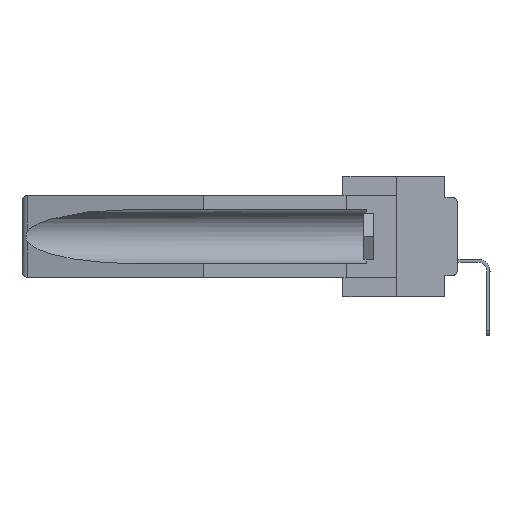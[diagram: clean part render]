
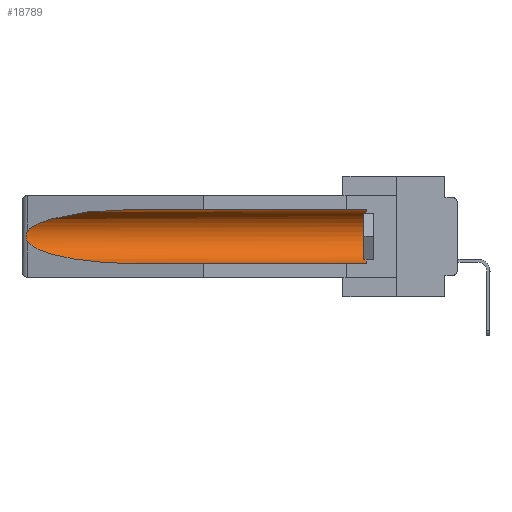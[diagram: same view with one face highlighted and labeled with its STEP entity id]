
A CAD part, left-side view. The second image highlights one B-rep face of the part: STEP entity #18789.
In plain terms, the highlighted cylindrical face has radius 2.857 mm (diameter 5.715 mm), a partial arc.
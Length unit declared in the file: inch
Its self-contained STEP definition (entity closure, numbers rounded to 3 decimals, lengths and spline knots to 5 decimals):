
#248 = DIRECTION ( 'NONE',  ( 0., 1., 0. ) ) ;
#819 = DIRECTION ( 'NONE',  ( 0., -1., 0. ) ) ;
#1037 = ORIENTED_EDGE ( 'NONE', *, *, #22426, .T. ) ;
#1324 = VECTOR ( 'NONE', #248, 39.37008 ) ;
#1703 = EDGE_LOOP ( 'NONE', ( #1764, #1037, #18259, #5178, #1854, #29031 ) ) ;
#1764 = ORIENTED_EDGE ( 'NONE', *, *, #3592, .T. ) ;
#1811 = CARTESIAN_POINT ( 'NONE',  ( 0.26537, 1.52718, -0.14972 ) ) ;
#1854 = ORIENTED_EDGE ( 'NONE', *, *, #24292, .T. ) ;
#1892 = AXIS2_PLACEMENT_3D ( 'NONE', #28931, #8678, #13623 ) ;
#2769 =( BOUNDED_CURVE ( )  B_SPLINE_CURVE ( 3, ( #29566, #17259, #4664, #7214 ),
 .UNSPECIFIED., .F., .F. ) 
 B_SPLINE_CURVE_WITH_KNOTS ( ( 4, 4 ),
 ( 0.1948, 1.5708 ),
 .UNSPECIFIED. ) 
 CURVE ( )  GEOMETRIC_REPRESENTATION_ITEM ( )  RATIONAL_B_SPLINE_CURVE ( ( 1., 0.848, 0.848, 1. ) ) 
 REPRESENTATION_ITEM ( '' )  );
#2864 = CARTESIAN_POINT ( 'NONE',  ( 0.26597, 1.52961, -0.15275 ) ) ;
#2960 = CARTESIAN_POINT ( 'NONE',  ( 0.2675, 1.53308, -0.17534 ) ) ;
#3379 = CARTESIAN_POINT ( 'NONE',  ( 0.26537, 1.52718, -0.14972 ) ) ;
#3592 = EDGE_CURVE ( 'NONE', #9058, #27754, #6649, .T. ) ;
#3792 = CARTESIAN_POINT ( 'NONE',  ( 0.2673, 1.53269, -0.17917 ) ) ;
#4254 = CARTESIAN_POINT ( 'NONE',  ( 0.155, 1.07973, -0.059 ) ) ;
#4664 = CARTESIAN_POINT ( 'NONE',  ( 0.21114, 1.30732, -0.284 ) ) ;
#4890 = CYLINDRICAL_SURFACE ( 'NONE', #1892, 0.1125 ) ;
#5091 = CIRCLE ( 'NONE', #12571, 0.1125 ) ;
#5178 = ORIENTED_EDGE ( 'NONE', *, *, #19157, .F. ) ;
#6057 = CARTESIAN_POINT ( 'NONE',  ( 0.155, 0.126, -0.1715 ) ) ;
#6424 = VERTEX_POINT ( 'NONE', #31843 ) ;
#6649 =( BOUNDED_CURVE ( )  B_SPLINE_CURVE ( 3, ( #4254, #21891, #22114, #1811 ),
 .UNSPECIFIED., .F., .F. ) 
 B_SPLINE_CURVE_WITH_KNOTS ( ( 4, 4 ),
 ( 4.71239, 6.08839 ),
 .UNSPECIFIED. ) 
 CURVE ( )  GEOMETRIC_REPRESENTATION_ITEM ( )  RATIONAL_B_SPLINE_CURVE ( ( 1., 0.848, 0.848, 1. ) ) 
 REPRESENTATION_ITEM ( '' )  );
#7214 = CARTESIAN_POINT ( 'NONE',  ( 0.155, 1.07973, -0.284 ) ) ;
#8256 = B_SPLINE_CURVE_WITH_KNOTS ( 'NONE', 3,
 ( #22686, #2864, #20324, #20540, #13003, #2960, #3792, #9309, #13583, #29938 ),
 .UNSPECIFIED., .F., .F.,
 ( 4, 2, 2, 2, 4 ),
 ( 0., 0.00029, 0.00058, 0.00087, 0.00117 ),
 .UNSPECIFIED. ) ;
#8678 = DIRECTION ( 'NONE',  ( 0., 1., 0. ) ) ;
#9058 = VERTEX_POINT ( 'NONE', #22231 ) ;
#9250 = CARTESIAN_POINT ( 'NONE',  ( 0.155, -0.30754, -0.059 ) ) ;
#9309 = CARTESIAN_POINT ( 'NONE',  ( 0.26655, 1.53094, -0.18657 ) ) ;
#9631 = LINE ( 'NONE', #12727, #1324 ) ;
#12571 = AXIS2_PLACEMENT_3D ( 'NONE', #6057, #819, #13618 ) ;
#12727 = CARTESIAN_POINT ( 'NONE',  ( 0.155, -0.30754, -0.284 ) ) ;
#13003 = CARTESIAN_POINT ( 'NONE',  ( 0.2675, 1.53308, -0.16763 ) ) ;
#13583 = CARTESIAN_POINT ( 'NONE',  ( 0.26597, 1.5296, -0.19026 ) ) ;
#13618 = DIRECTION ( 'NONE',  ( 0., 0., 1. ) ) ;
#13623 = DIRECTION ( 'NONE',  ( 0., 0., 1. ) ) ;
#13958 = FACE_OUTER_BOUND ( 'NONE', #1703, .T. ) ;
#17007 = CARTESIAN_POINT ( 'NONE',  ( 0.155, 0.126, -0.284 ) ) ;
#17259 = CARTESIAN_POINT ( 'NONE',  ( 0.25451, 1.48313, -0.24835 ) ) ;
#18259 = ORIENTED_EDGE ( 'NONE', *, *, #26882, .T. ) ;
#18296 = VERTEX_POINT ( 'NONE', #17007 ) ;
#18789 = ADVANCED_FACE ( 'NONE', ( #13958 ), #4890, .F. ) ;
#19157 = EDGE_CURVE ( 'NONE', #18296, #25073, #9631, .T. ) ;
#19195 = VERTEX_POINT ( 'NONE', #25517 ) ;
#19422 = DIRECTION ( 'NONE',  ( 0., 1., 0. ) ) ;
#19493 = EDGE_CURVE ( 'NONE', #6424, #9058, #23428, .T. ) ;
#20324 = CARTESIAN_POINT ( 'NONE',  ( 0.26654, 1.53092, -0.15636 ) ) ;
#20540 = CARTESIAN_POINT ( 'NONE',  ( 0.2673, 1.5327, -0.16383 ) ) ;
#21891 = CARTESIAN_POINT ( 'NONE',  ( 0.21114, 1.30732, -0.059 ) ) ;
#22114 = CARTESIAN_POINT ( 'NONE',  ( 0.25451, 1.48313, -0.09465 ) ) ;
#22231 = CARTESIAN_POINT ( 'NONE',  ( 0.155, 1.07973, -0.059 ) ) ;
#22426 = EDGE_CURVE ( 'NONE', #27754, #19195, #8256, .T. ) ;
#22686 = CARTESIAN_POINT ( 'NONE',  ( 0.26537, 1.52718, -0.14972 ) ) ;
#23428 = LINE ( 'NONE', #9250, #30496 ) ;
#24292 = EDGE_CURVE ( 'NONE', #18296, #6424, #5091, .T. ) ;
#25073 = VERTEX_POINT ( 'NONE', #26585 ) ;
#25517 = CARTESIAN_POINT ( 'NONE',  ( 0.26537, 1.52718, -0.19328 ) ) ;
#26585 = CARTESIAN_POINT ( 'NONE',  ( 0.155, 1.07973, -0.284 ) ) ;
#26882 = EDGE_CURVE ( 'NONE', #19195, #25073, #2769, .T. ) ;
#27754 = VERTEX_POINT ( 'NONE', #3379 ) ;
#28931 = CARTESIAN_POINT ( 'NONE',  ( 0.155, -0.30754, -0.1715 ) ) ;
#29031 = ORIENTED_EDGE ( 'NONE', *, *, #19493, .T. ) ;
#29566 = CARTESIAN_POINT ( 'NONE',  ( 0.26537, 1.52718, -0.19328 ) ) ;
#29938 = CARTESIAN_POINT ( 'NONE',  ( 0.26537, 1.52718, -0.19328 ) ) ;
#30496 = VECTOR ( 'NONE', #19422, 39.37008 ) ;
#31843 = CARTESIAN_POINT ( 'NONE',  ( 0.155, 0.126, -0.059 ) ) ;
